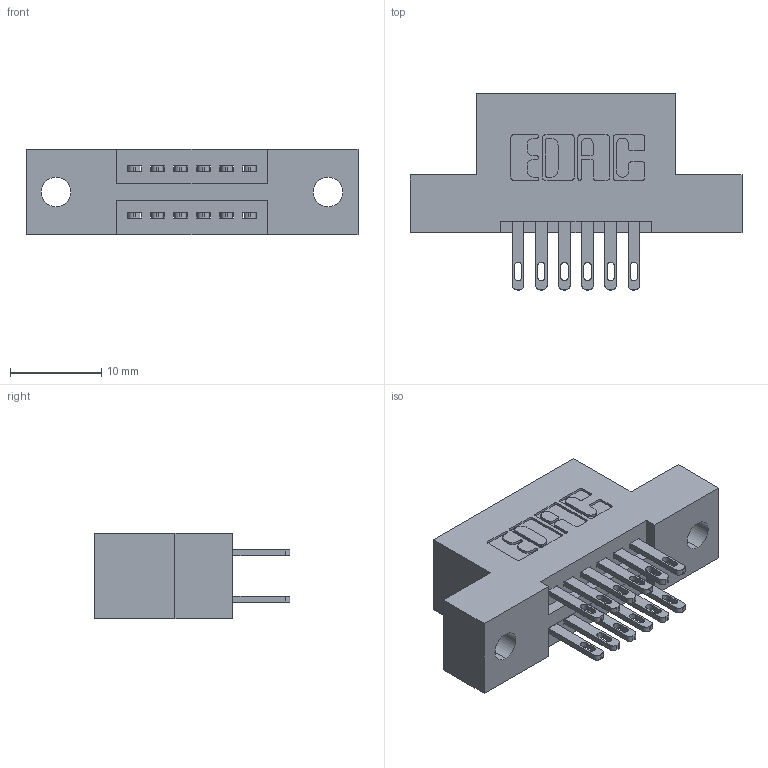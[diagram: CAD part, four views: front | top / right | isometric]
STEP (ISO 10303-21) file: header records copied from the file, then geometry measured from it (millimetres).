
FILE_DESCRIPTION (( 'STEP AP203' ), '1' );
FILE_NAME ('895-012-500-202.STEP', '2020-09-25T01:12:52', ( '' ), ( '' ), 'SwSTEP 2.0', 'SolidWorks 2020', '' );
FILE_SCHEMA (( 'CONFIG_CONTROL_DESIGN' ));
Length unit declared in the file: inch
Products named in the file (3): 845 Part_Flush Mounting Lugs - 0.128 Dia; 895-012-500-202; 345-292-001_345-293-100
Assembly tree (13 placements, depth 2):
  895-012-500-202
    845 Part_Flush Mounting Lugs - 0.128 Dia
    345-292-001_345-293-100  x12
Bounding box: 36.45 x 21.51 x 9.4 mm (x, y, z)
Volume: 3206.5 mm3; surface area: 3892.2 mm2
Topology: 13 solids, 13 shells, 678 faces, 2033 edges, 1354 vertices
Faces by surface type: plane 404, cylinder 274
Entity records: 9487 total; most frequent: CARTESIAN_POINT 1624, ORIENTED_EDGE 1558, DIRECTION 1479, EDGE_CURVE 779, LINE 619, VECTOR 619, VERTEX_POINT 518, AXIS2_PLACEMENT_3D 430
